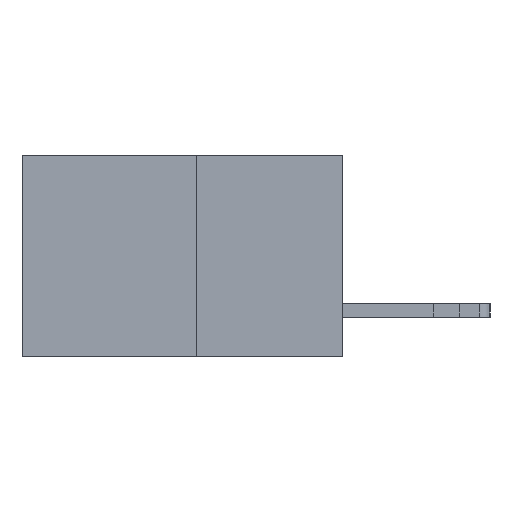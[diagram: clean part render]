
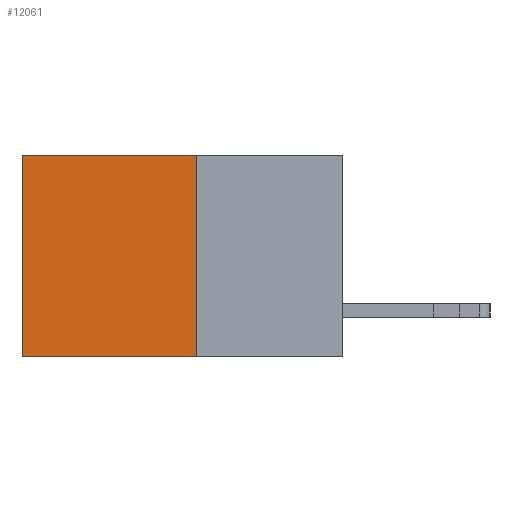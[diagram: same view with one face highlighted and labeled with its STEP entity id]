
A CAD part, left-side view. The second image highlights one B-rep face of the part: STEP entity #12061.
In plain terms, the highlighted planar face has unit normal (-1, 0, 0).
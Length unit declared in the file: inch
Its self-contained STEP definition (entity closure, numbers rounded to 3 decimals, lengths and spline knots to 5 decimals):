
#212 = ORIENTED_EDGE ( 'NONE', *, *, #4349, .T. ) ;
#348 = LINE ( 'NONE', #13879, #702 ) ;
#369 = CARTESIAN_POINT ( 'NONE',  ( 0.277, 0.27, -0.37 ) ) ;
#702 = VECTOR ( 'NONE', #6046, 39.37008 ) ;
#793 = VERTEX_POINT ( 'NONE', #369 ) ;
#1760 = ORIENTED_EDGE ( 'NONE', *, *, #12246, .F. ) ;
#1952 = CARTESIAN_POINT ( 'NONE',  ( 0.277, 0.27, 0. ) ) ;
#2507 = DIRECTION ( 'NONE',  ( 0., 1., 0. ) ) ;
#2586 = FACE_OUTER_BOUND ( 'NONE', #12406, .T. ) ;
#2976 = LINE ( 'NONE', #5978, #12045 ) ;
#3625 = LINE ( 'NONE', #1952, #12334 ) ;
#4254 = LINE ( 'NONE', #7495, #4611 ) ;
#4316 = ORIENTED_EDGE ( 'NONE', *, *, #10067, .F. ) ;
#4349 = EDGE_CURVE ( 'NONE', #6729, #14195, #4254, .T. ) ;
#4611 = VECTOR ( 'NONE', #7445, 39.37008 ) ;
#5643 = DIRECTION ( 'NONE',  ( 1., 0., 0. ) ) ;
#5864 = VERTEX_POINT ( 'NONE', #12853 ) ;
#5978 = CARTESIAN_POINT ( 'NONE',  ( 0.277, 0.27, -0.37 ) ) ;
#6046 = DIRECTION ( 'NONE',  ( 0., 0., -1. ) ) ;
#6729 = VERTEX_POINT ( 'NONE', #8730 ) ;
#7445 = DIRECTION ( 'NONE',  ( 0., 0., -1. ) ) ;
#7495 = CARTESIAN_POINT ( 'NONE',  ( 0.277, 0.59, -0.37 ) ) ;
#8730 = CARTESIAN_POINT ( 'NONE',  ( 0.277, 0.59, 0. ) ) ;
#9515 = CARTESIAN_POINT ( 'NONE',  ( 0.277, 0.59, -0.37 ) ) ;
#9853 = ORIENTED_EDGE ( 'NONE', *, *, #14318, .T. ) ;
#9887 = AXIS2_PLACEMENT_3D ( 'NONE', #14535, #5643, #13518 ) ;
#10067 = EDGE_CURVE ( 'NONE', #5864, #793, #348, .T. ) ;
#12045 = VECTOR ( 'NONE', #2507, 39.37008 ) ;
#12061 = ADVANCED_FACE ( 'NONE', ( #2586 ), #13470, .F. ) ;
#12246 = EDGE_CURVE ( 'NONE', #793, #14195, #2976, .T. ) ;
#12334 = VECTOR ( 'NONE', #13239, 39.37008 ) ;
#12406 = EDGE_LOOP ( 'NONE', ( #212, #1760, #4316, #9853 ) ) ;
#12853 = CARTESIAN_POINT ( 'NONE',  ( 0.277, 0.27, 0. ) ) ;
#13239 = DIRECTION ( 'NONE',  ( 0., 1., 0. ) ) ;
#13470 = PLANE ( 'NONE',  #9887 ) ;
#13518 = DIRECTION ( 'NONE',  ( 0., 0., -1. ) ) ;
#13879 = CARTESIAN_POINT ( 'NONE',  ( 0.277, 0.27, -0.37 ) ) ;
#14195 = VERTEX_POINT ( 'NONE', #9515 ) ;
#14318 = EDGE_CURVE ( 'NONE', #5864, #6729, #3625, .T. ) ;
#14535 = CARTESIAN_POINT ( 'NONE',  ( 0.277, 0.27, -0.37 ) ) ;
